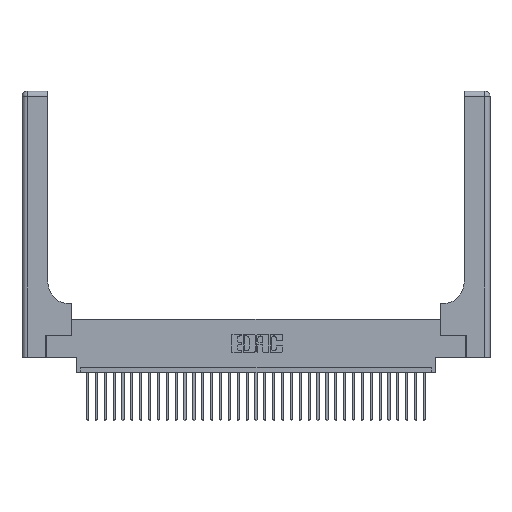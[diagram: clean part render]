
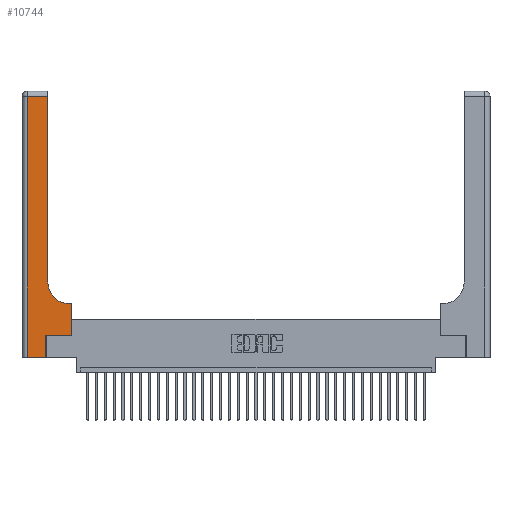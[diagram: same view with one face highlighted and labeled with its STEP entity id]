
A CAD part, top view. The second image highlights one B-rep face of the part: STEP entity #10744.
In plain terms, the highlighted planar face has unit normal (0, 0, 1).
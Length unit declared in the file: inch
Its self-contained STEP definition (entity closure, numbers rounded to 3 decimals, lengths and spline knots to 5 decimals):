
#712 = DIRECTION ( 'NONE',  ( 1., 0., 0. ) ) ;
#862 = CARTESIAN_POINT ( 'NONE',  ( 0.2915, 3., 0.37 ) ) ;
#1333 = CARTESIAN_POINT ( 'NONE',  ( 0.5585, 0.25, 0.37 ) ) ;
#1449 = CARTESIAN_POINT ( 'NONE',  ( 0.269, 0.25, 0.37 ) ) ;
#2245 = ORIENTED_EDGE ( 'NONE', *, *, #31922, .T. ) ;
#2325 = VECTOR ( 'NONE', #20151, 39.37008 ) ;
#2348 = CARTESIAN_POINT ( 'NONE',  ( 0.5415, 0.85, 0.37 ) ) ;
#3647 = DIRECTION ( 'NONE',  ( 1., 0., 0. ) ) ;
#3803 = EDGE_CURVE ( 'NONE', #30023, #8324, #11478, .T. ) ;
#5581 = ORIENTED_EDGE ( 'NONE', *, *, #22629, .T. ) ;
#6211 = CARTESIAN_POINT ( 'NONE',  ( 0.5415, 0.6, 0.37 ) ) ;
#7443 = CARTESIAN_POINT ( 'NONE',  ( 0., 3., 0.37 ) ) ;
#7499 = LINE ( 'NONE', #11380, #21026 ) ;
#7649 = VERTEX_POINT ( 'NONE', #20559 ) ;
#7687 = VERTEX_POINT ( 'NONE', #11988 ) ;
#7927 = EDGE_CURVE ( 'NONE', #10288, #7649, #8450, .T. ) ;
#8324 = VERTEX_POINT ( 'NONE', #6211 ) ;
#8450 = LINE ( 'NONE', #28311, #13963 ) ;
#8533 = VECTOR ( 'NONE', #26675, 39.37008 ) ;
#10077 = AXIS2_PLACEMENT_3D ( 'NONE', #7443, #34344, #29004 ) ;
#10288 = VERTEX_POINT ( 'NONE', #32476 ) ;
#10736 = DIRECTION ( 'NONE',  ( 0., 1., 0. ) ) ;
#10744 = ADVANCED_FACE ( 'NONE', ( #11224 ), #23677, .F. ) ;
#11224 = FACE_OUTER_BOUND ( 'NONE', #34361, .T. ) ;
#11380 = CARTESIAN_POINT ( 'NONE',  ( 0.269, 0., 0.37 ) ) ;
#11478 = LINE ( 'NONE', #13430, #23398 ) ;
#11988 = CARTESIAN_POINT ( 'NONE',  ( 0.2915, 0.85, 0.37 ) ) ;
#12565 = VECTOR ( 'NONE', #13942, 39.37008 ) ;
#13430 = CARTESIAN_POINT ( 'NONE',  ( 0.2915, 0.6, 0.37 ) ) ;
#13942 = DIRECTION ( 'NONE',  ( 0., -1., 0. ) ) ;
#13963 = VECTOR ( 'NONE', #712, 39.37008 ) ;
#14757 = CARTESIAN_POINT ( 'NONE',  ( 0.2915, 2.94, 0.37 ) ) ;
#15029 = LINE ( 'NONE', #862, #2325 ) ;
#15094 = ORIENTED_EDGE ( 'NONE', *, *, #3803, .T. ) ;
#16358 = DIRECTION ( 'NONE',  ( 0., 1., 0. ) ) ;
#16647 = LINE ( 'NONE', #1449, #28609 ) ;
#17510 = AXIS2_PLACEMENT_3D ( 'NONE', #2348, #26678, #29815 ) ;
#17683 = ORIENTED_EDGE ( 'NONE', *, *, #21820, .T. ) ;
#18032 = LINE ( 'NONE', #27593, #12565 ) ;
#18596 = ORIENTED_EDGE ( 'NONE', *, *, #27674, .T. ) ;
#18906 = ORIENTED_EDGE ( 'NONE', *, *, #26490, .T. ) ;
#20151 = DIRECTION ( 'NONE',  ( 0., 1., 0. ) ) ;
#20559 = CARTESIAN_POINT ( 'NONE',  ( 0.269, 0., 0.37 ) ) ;
#21026 = VECTOR ( 'NONE', #16358, 39.37008 ) ;
#21820 = EDGE_CURVE ( 'NONE', #7649, #25168, #7499, .T. ) ;
#22629 = EDGE_CURVE ( 'NONE', #25168, #26254, #16647, .T. ) ;
#22771 = VECTOR ( 'NONE', #10736, 39.37008 ) ;
#23398 = VECTOR ( 'NONE', #32390, 39.37008 ) ;
#23576 = CARTESIAN_POINT ( 'NONE',  ( 0., 2.94, 0.37 ) ) ;
#23677 = PLANE ( 'NONE',  #10077 ) ;
#23886 = LINE ( 'NONE', #23576, #8533 ) ;
#25168 = VERTEX_POINT ( 'NONE', #26528 ) ;
#25478 = EDGE_CURVE ( 'NONE', #7687, #29794, #15029, .T. ) ;
#26254 = VERTEX_POINT ( 'NONE', #1333 ) ;
#26490 = EDGE_CURVE ( 'NONE', #29794, #30705, #23886, .T. ) ;
#26528 = CARTESIAN_POINT ( 'NONE',  ( 0.269, 0.25, 0.37 ) ) ;
#26675 = DIRECTION ( 'NONE',  ( -1., 0., 0. ) ) ;
#26678 = DIRECTION ( 'NONE',  ( 0., 0., -1. ) ) ;
#27593 = CARTESIAN_POINT ( 'NONE',  ( 0.06, 3., 0.37 ) ) ;
#27674 = EDGE_CURVE ( 'NONE', #8324, #7687, #29306, .T. ) ;
#27868 = LINE ( 'NONE', #32091, #22771 ) ;
#28311 = CARTESIAN_POINT ( 'NONE',  ( 0., 0., 0.37 ) ) ;
#28609 = VECTOR ( 'NONE', #3647, 39.37008 ) ;
#29004 = DIRECTION ( 'NONE',  ( -1., 0., 0. ) ) ;
#29306 = CIRCLE ( 'NONE', #17510, 0.25 ) ;
#29460 = CARTESIAN_POINT ( 'NONE',  ( 0.5585, 0.6, 0.37 ) ) ;
#29534 = EDGE_CURVE ( 'NONE', #26254, #30023, #27868, .T. ) ;
#29794 = VERTEX_POINT ( 'NONE', #14757 ) ;
#29815 = DIRECTION ( 'NONE',  ( 1., 0., 0. ) ) ;
#29828 = ORIENTED_EDGE ( 'NONE', *, *, #25478, .T. ) ;
#29929 = CARTESIAN_POINT ( 'NONE',  ( 0.06, 2.94, 0.37 ) ) ;
#30023 = VERTEX_POINT ( 'NONE', #29460 ) ;
#30705 = VERTEX_POINT ( 'NONE', #29929 ) ;
#31212 = ORIENTED_EDGE ( 'NONE', *, *, #29534, .T. ) ;
#31922 = EDGE_CURVE ( 'NONE', #30705, #10288, #18032, .T. ) ;
#32091 = CARTESIAN_POINT ( 'NONE',  ( 0.5585, 0.25, 0.37 ) ) ;
#32390 = DIRECTION ( 'NONE',  ( -1., 0., 0. ) ) ;
#32476 = CARTESIAN_POINT ( 'NONE',  ( 0.06, 0., 0.37 ) ) ;
#34344 = DIRECTION ( 'NONE',  ( 0., 0., -1. ) ) ;
#34361 = EDGE_LOOP ( 'NONE', ( #29828, #18906, #2245, #34767, #17683, #5581, #31212, #15094, #18596 ) ) ;
#34767 = ORIENTED_EDGE ( 'NONE', *, *, #7927, .T. ) ;
